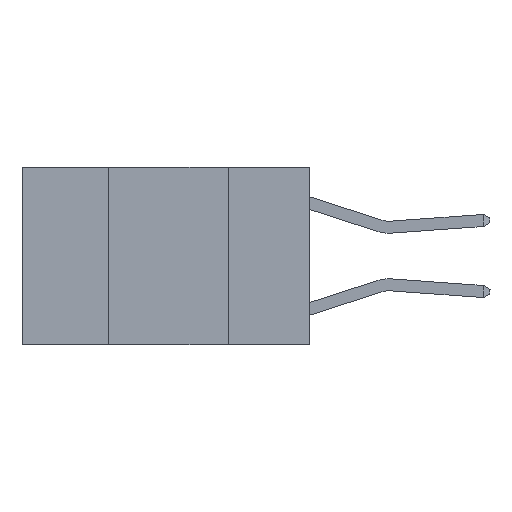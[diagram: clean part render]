
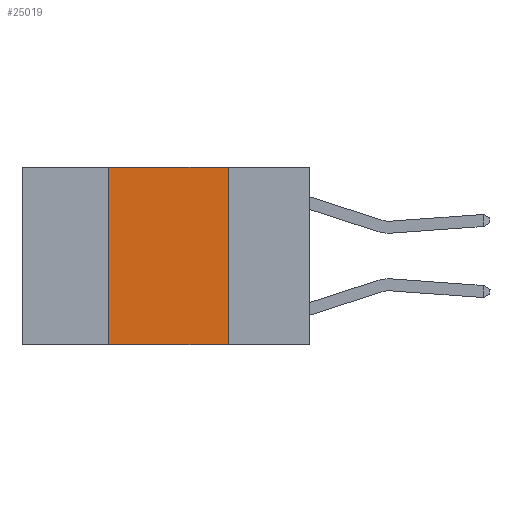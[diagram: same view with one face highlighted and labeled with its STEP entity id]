
A CAD part, left-side view. The second image highlights one B-rep face of the part: STEP entity #25019.
In plain terms, the highlighted planar face has unit normal (-1, 0, 0).
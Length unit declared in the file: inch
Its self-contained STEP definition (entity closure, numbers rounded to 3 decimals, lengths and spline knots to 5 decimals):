
#786 = LINE ( 'NONE', #8426, #13175 ) ;
#1499 = FACE_OUTER_BOUND ( 'NONE', #24327, .T. ) ;
#1611 = CARTESIAN_POINT ( 'NONE',  ( 0., 0.17, -0.37 ) ) ;
#3076 = CARTESIAN_POINT ( 'NONE',  ( 0., 0.17, 0. ) ) ;
#3967 = EDGE_CURVE ( 'NONE', #19256, #6467, #17844, .T. ) ;
#5750 = VECTOR ( 'NONE', #27381, 39.37008 ) ;
#6231 = VECTOR ( 'NONE', #10712, 39.37008 ) ;
#6240 = ORIENTED_EDGE ( 'NONE', *, *, #27906, .F. ) ;
#6467 = VERTEX_POINT ( 'NONE', #1611 ) ;
#8274 = DIRECTION ( 'NONE',  ( 1., 0., 0. ) ) ;
#8426 = CARTESIAN_POINT ( 'NONE',  ( 0., 0.6, -0.37 ) ) ;
#9152 = CARTESIAN_POINT ( 'NONE',  ( 0., 0.42, 0. ) ) ;
#10712 = DIRECTION ( 'NONE',  ( 0., 0., -1. ) ) ;
#10854 = AXIS2_PLACEMENT_3D ( 'NONE', #15187, #8274, #24425 ) ;
#11642 = VECTOR ( 'NONE', #16623, 39.37008 ) ;
#11963 = LINE ( 'NONE', #9152, #5750 ) ;
#12376 = LINE ( 'NONE', #14294, #11642 ) ;
#13175 = VECTOR ( 'NONE', #24560, 39.37008 ) ;
#14158 = EDGE_CURVE ( 'NONE', #25464, #6467, #786, .T. ) ;
#14294 = CARTESIAN_POINT ( 'NONE',  ( 0., 0.6, 0. ) ) ;
#14618 = CARTESIAN_POINT ( 'NONE',  ( 0., 0.42, 0. ) ) ;
#15187 = CARTESIAN_POINT ( 'NONE',  ( 0., 0.6, 0. ) ) ;
#16623 = DIRECTION ( 'NONE',  ( 0., -1., 0. ) ) ;
#16665 = CARTESIAN_POINT ( 'NONE',  ( 0., 0.42, -0.37 ) ) ;
#17844 = LINE ( 'NONE', #24510, #6231 ) ;
#18384 = ORIENTED_EDGE ( 'NONE', *, *, #20950, .F. ) ;
#19256 = VERTEX_POINT ( 'NONE', #3076 ) ;
#20602 = ORIENTED_EDGE ( 'NONE', *, *, #14158, .T. ) ;
#20950 = EDGE_CURVE ( 'NONE', #25464, #21171, #11963, .T. ) ;
#21171 = VERTEX_POINT ( 'NONE', #14618 ) ;
#24327 = EDGE_LOOP ( 'NONE', ( #25393, #6240, #18384, #20602 ) ) ;
#24425 = DIRECTION ( 'NONE',  ( 0., 0., -1. ) ) ;
#24510 = CARTESIAN_POINT ( 'NONE',  ( 0., 0.17, 0. ) ) ;
#24560 = DIRECTION ( 'NONE',  ( 0., -1., 0. ) ) ;
#25019 = ADVANCED_FACE ( 'NONE', ( #1499 ), #28794, .F. ) ;
#25393 = ORIENTED_EDGE ( 'NONE', *, *, #3967, .F. ) ;
#25464 = VERTEX_POINT ( 'NONE', #16665 ) ;
#27381 = DIRECTION ( 'NONE',  ( 0., 0., 1. ) ) ;
#27906 = EDGE_CURVE ( 'NONE', #21171, #19256, #12376, .T. ) ;
#28794 = PLANE ( 'NONE',  #10854 ) ;
